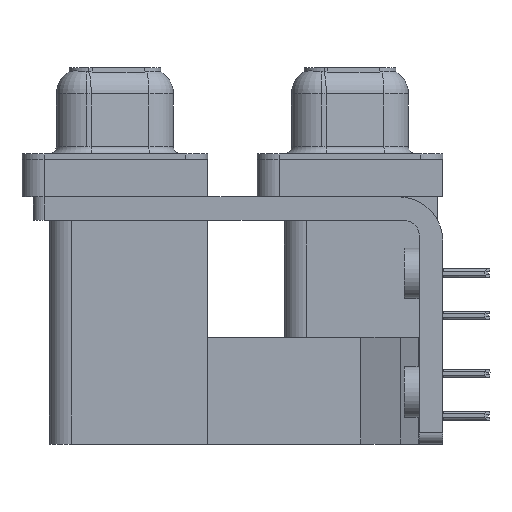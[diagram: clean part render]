
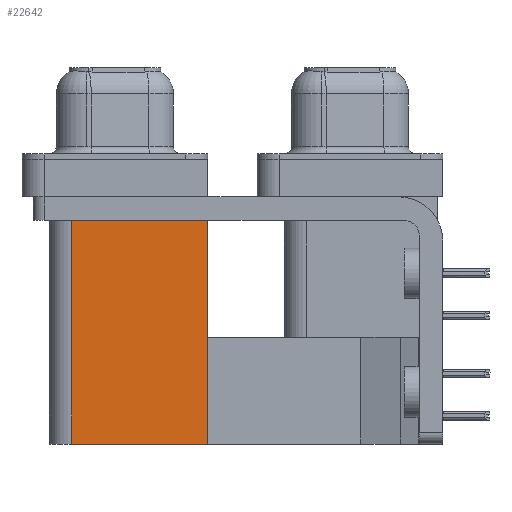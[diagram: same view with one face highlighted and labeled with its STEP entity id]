
A CAD part, left-side view. The second image highlights one B-rep face of the part: STEP entity #22642.
In plain terms, the highlighted planar face has unit normal (-1, 0, 0).
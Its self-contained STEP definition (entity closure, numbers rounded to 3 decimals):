
#1084 = AXIS2_PLACEMENT_3D ( 'NONE', #5157, #4495, #31960 ) ;
#2678 = CARTESIAN_POINT ( 'NONE',  ( 3.79, 9.6, -2.5 ) ) ;
#3484 = EDGE_CURVE ( 'NONE', #32483, #4698, #18620, .T. ) ;
#3530 = ORIENTED_EDGE ( 'NONE', *, *, #37514, .T. ) ;
#4495 = DIRECTION ( 'NONE',  ( 1., 0., 0. ) ) ;
#4698 = VERTEX_POINT ( 'NONE', #20980 ) ;
#4721 = EDGE_CURVE ( 'NONE', #32483, #39241, #13779, .T. ) ;
#5157 = CARTESIAN_POINT ( 'NONE',  ( 3.79, 9.6, -19.2 ) ) ;
#5646 = VERTEX_POINT ( 'NONE', #25943 ) ;
#9406 = VECTOR ( 'NONE', #35318, 1000. ) ;
#9939 = ORIENTED_EDGE ( 'NONE', *, *, #3484, .T. ) ;
#10591 = LINE ( 'NONE', #38291, #20535 ) ;
#12148 = FACE_OUTER_BOUND ( 'NONE', #19674, .T. ) ;
#12818 = DIRECTION ( 'NONE',  ( 0., 1., 0. ) ) ;
#13776 = VECTOR ( 'NONE', #31791, 1000. ) ;
#13779 = LINE ( 'NONE', #21421, #13776 ) ;
#15429 = VECTOR ( 'NONE', #12818, 1000. ) ;
#16776 = ORIENTED_EDGE ( 'NONE', *, *, #4721, .F. ) ;
#18620 = LINE ( 'NONE', #39375, #9406 ) ;
#19674 = EDGE_LOOP ( 'NONE', ( #3530, #33476, #16776, #9939 ) ) ;
#20535 = VECTOR ( 'NONE', #30619, 1000. ) ;
#20980 = CARTESIAN_POINT ( 'NONE',  ( 3.79, 9.6, -2.5 ) ) ;
#21335 = EDGE_CURVE ( 'NONE', #39241, #5646, #10591, .T. ) ;
#21421 = CARTESIAN_POINT ( 'NONE',  ( 3.79, 9.6, -19.2 ) ) ;
#21817 = PLANE ( 'NONE',  #1084 ) ;
#22642 = ADVANCED_FACE ( 'NONE', ( #12148 ), #21817, .F. ) ;
#23361 = LINE ( 'NONE', #2678, #15429 ) ;
#25943 = CARTESIAN_POINT ( 'NONE',  ( 3.79, 18.8, -2.5 ) ) ;
#30619 = DIRECTION ( 'NONE',  ( 0., 0., 1. ) ) ;
#31791 = DIRECTION ( 'NONE',  ( 0., 1., 0. ) ) ;
#31960 = DIRECTION ( 'NONE',  ( 0., 1., 0. ) ) ;
#32483 = VERTEX_POINT ( 'NONE', #36705 ) ;
#33476 = ORIENTED_EDGE ( 'NONE', *, *, #21335, .F. ) ;
#35318 = DIRECTION ( 'NONE',  ( 0., 0., 1. ) ) ;
#36705 = CARTESIAN_POINT ( 'NONE',  ( 3.79, 9.6, -19.2 ) ) ;
#37514 = EDGE_CURVE ( 'NONE', #4698, #5646, #23361, .T. ) ;
#38291 = CARTESIAN_POINT ( 'NONE',  ( 3.79, 18.8, -19.2 ) ) ;
#38430 = CARTESIAN_POINT ( 'NONE',  ( 3.79, 18.8, -19.2 ) ) ;
#39241 = VERTEX_POINT ( 'NONE', #38430 ) ;
#39375 = CARTESIAN_POINT ( 'NONE',  ( 3.79, 9.6, -19.2 ) ) ;
